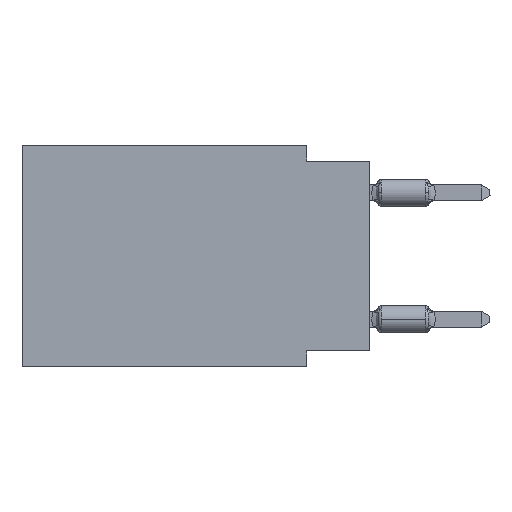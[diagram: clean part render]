
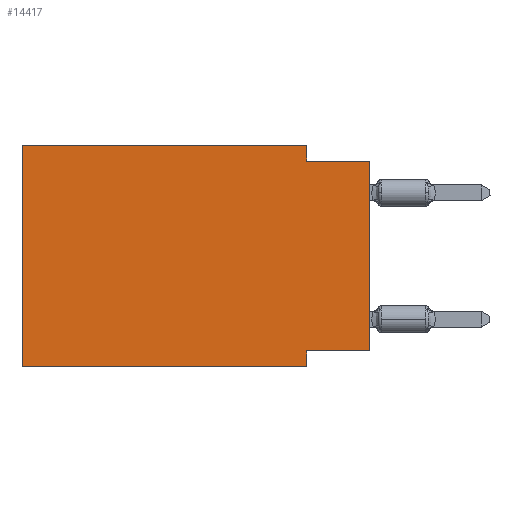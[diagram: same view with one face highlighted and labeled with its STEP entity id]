
A CAD part, left-side view. The second image highlights one B-rep face of the part: STEP entity #14417.
In plain terms, the highlighted planar face has unit normal (-1, 0, 0).
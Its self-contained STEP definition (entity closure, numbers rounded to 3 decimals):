
#1143 = LINE ( 'NONE', #13464, #19282 ) ;
#1205 = VECTOR ( 'NONE', #23843, 1000. ) ;
#1312 = EDGE_CURVE ( 'NONE', #17247, #11204, #5632, .T. ) ;
#1331 = FACE_OUTER_BOUND ( 'NONE', #2568, .T. ) ;
#1351 = DIRECTION ( 'NONE',  ( 0., 0., -1. ) ) ;
#2187 = EDGE_CURVE ( 'NONE', #16493, #25247, #1143, .T. ) ;
#2568 = EDGE_LOOP ( 'NONE', ( #17949, #18950, #25958, #21592, #18141, #7656, #21415, #5980 ) ) ;
#2683 = LINE ( 'NONE', #15393, #1205 ) ;
#2715 = CARTESIAN_POINT ( 'NONE',  ( 0., 2.54, -8.89 ) ) ;
#2994 = DIRECTION ( 'NONE',  ( 0., 1., 0. ) ) ;
#3551 = LINE ( 'NONE', #6159, #11476 ) ;
#3684 = CARTESIAN_POINT ( 'NONE',  ( 0., 13.97, 0. ) ) ;
#3841 = VECTOR ( 'NONE', #1351, 1000. ) ;
#4521 = LINE ( 'NONE', #4940, #17291 ) ;
#4642 = DIRECTION ( 'NONE',  ( 0., 0., 1. ) ) ;
#4940 = CARTESIAN_POINT ( 'NONE',  ( 0., 0., -8.255 ) ) ;
#5103 = CARTESIAN_POINT ( 'NONE',  ( 0., 2.54, 0. ) ) ;
#5632 = LINE ( 'NONE', #5103, #3841 ) ;
#5775 = CARTESIAN_POINT ( 'NONE',  ( 0., 0., -0.635 ) ) ;
#5881 = DIRECTION ( 'NONE',  ( 0., 0., -1. ) ) ;
#5980 = ORIENTED_EDGE ( 'NONE', *, *, #24501, .F. ) ;
#6159 = CARTESIAN_POINT ( 'NONE',  ( 0., 2.54, -8.89 ) ) ;
#6760 = CARTESIAN_POINT ( 'NONE',  ( 0., 0., -0.635 ) ) ;
#7656 = ORIENTED_EDGE ( 'NONE', *, *, #18266, .T. ) ;
#9589 = DIRECTION ( 'NONE',  ( 0., 0., 1. ) ) ;
#10044 = DIRECTION ( 'NONE',  ( 0., 0., -1. ) ) ;
#11204 = VERTEX_POINT ( 'NONE', #16798 ) ;
#11298 = LINE ( 'NONE', #15595, #17456 ) ;
#11411 = VECTOR ( 'NONE', #4642, 1000. ) ;
#11476 = VECTOR ( 'NONE', #5881, 1000. ) ;
#11978 = CARTESIAN_POINT ( 'NONE',  ( 0., 13.97, -8.89 ) ) ;
#13464 = CARTESIAN_POINT ( 'NONE',  ( 0., 0., 0. ) ) ;
#14417 = ADVANCED_FACE ( 'NONE', ( #1331 ), #24584, .F. ) ;
#15111 = EDGE_CURVE ( 'NONE', #17195, #17247, #2683, .T. ) ;
#15393 = CARTESIAN_POINT ( 'NONE',  ( 0., 13.97, 0. ) ) ;
#15595 = CARTESIAN_POINT ( 'NONE',  ( 0., 13.97, -8.89 ) ) ;
#16243 = VECTOR ( 'NONE', #25528, 1000. ) ;
#16493 = VERTEX_POINT ( 'NONE', #19528 ) ;
#16798 = CARTESIAN_POINT ( 'NONE',  ( 0., 2.54, -0.635 ) ) ;
#17195 = VERTEX_POINT ( 'NONE', #23020 ) ;
#17247 = VERTEX_POINT ( 'NONE', #20803 ) ;
#17291 = VECTOR ( 'NONE', #2994, 1000. ) ;
#17366 = LINE ( 'NONE', #21232, #11411 ) ;
#17456 = VECTOR ( 'NONE', #20036, 1000. ) ;
#17949 = ORIENTED_EDGE ( 'NONE', *, *, #2187, .T. ) ;
#18141 = ORIENTED_EDGE ( 'NONE', *, *, #22425, .F. ) ;
#18266 = EDGE_CURVE ( 'NONE', #22285, #18426, #11298, .T. ) ;
#18426 = VERTEX_POINT ( 'NONE', #2715 ) ;
#18950 = ORIENTED_EDGE ( 'NONE', *, *, #20518, .F. ) ;
#19282 = VECTOR ( 'NONE', #9589, 1000. ) ;
#19528 = CARTESIAN_POINT ( 'NONE',  ( 0., 0., -8.255 ) ) ;
#19598 = CARTESIAN_POINT ( 'NONE',  ( 0., 2.54, -8.255 ) ) ;
#19632 = AXIS2_PLACEMENT_3D ( 'NONE', #3684, #22920, #10044 ) ;
#20036 = DIRECTION ( 'NONE',  ( 0., -1., 0. ) ) ;
#20518 = EDGE_CURVE ( 'NONE', #11204, #25247, #24873, .T. ) ;
#20803 = CARTESIAN_POINT ( 'NONE',  ( 0., 2.54, 0. ) ) ;
#21232 = CARTESIAN_POINT ( 'NONE',  ( 0., 13.97, 0. ) ) ;
#21415 = ORIENTED_EDGE ( 'NONE', *, *, #23526, .F. ) ;
#21592 = ORIENTED_EDGE ( 'NONE', *, *, #15111, .F. ) ;
#22285 = VERTEX_POINT ( 'NONE', #11978 ) ;
#22425 = EDGE_CURVE ( 'NONE', #22285, #17195, #17366, .T. ) ;
#22920 = DIRECTION ( 'NONE',  ( 1., 0., 0. ) ) ;
#23020 = CARTESIAN_POINT ( 'NONE',  ( 0., 13.97, 0. ) ) ;
#23526 = EDGE_CURVE ( 'NONE', #23666, #18426, #3551, .T. ) ;
#23666 = VERTEX_POINT ( 'NONE', #19598 ) ;
#23843 = DIRECTION ( 'NONE',  ( 0., -1., 0. ) ) ;
#24501 = EDGE_CURVE ( 'NONE', #16493, #23666, #4521, .T. ) ;
#24584 = PLANE ( 'NONE',  #19632 ) ;
#24873 = LINE ( 'NONE', #5775, #16243 ) ;
#25247 = VERTEX_POINT ( 'NONE', #6760 ) ;
#25528 = DIRECTION ( 'NONE',  ( 0., -1., 0. ) ) ;
#25958 = ORIENTED_EDGE ( 'NONE', *, *, #1312, .F. ) ;
